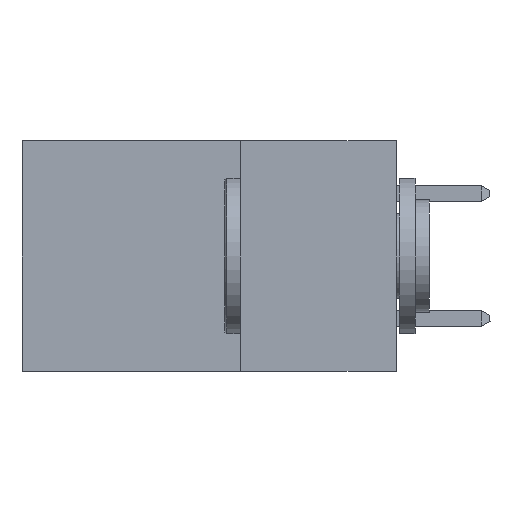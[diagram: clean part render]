
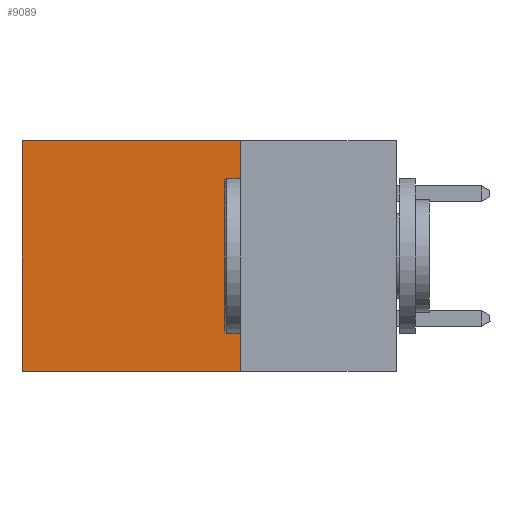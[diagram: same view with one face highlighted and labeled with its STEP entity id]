
A CAD part, left-side view. The second image highlights one B-rep face of the part: STEP entity #9089.
In plain terms, the highlighted planar face has unit normal (-1, 0, 0).
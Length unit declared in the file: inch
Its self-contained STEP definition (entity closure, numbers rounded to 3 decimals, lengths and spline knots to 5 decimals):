
#86 = ORIENTED_EDGE ( 'NONE', *, *, #2505, .F. ) ;
#507 = PLANE ( 'NONE',  #6340 ) ;
#797 = VECTOR ( 'NONE', #9953, 39.37008 ) ;
#891 = CARTESIAN_POINT ( 'NONE',  ( 0.2615, 0.25, -0.37 ) ) ;
#1397 = EDGE_CURVE ( 'NONE', #5189, #5558, #2477, .T. ) ;
#2044 = DIRECTION ( 'NONE',  ( 1., 0., 0. ) ) ;
#2215 = VECTOR ( 'NONE', #5669, 39.37008 ) ;
#2477 = LINE ( 'NONE', #4899, #2215 ) ;
#2505 = EDGE_CURVE ( 'NONE', #5189, #9576, #9101, .T. ) ;
#2617 = LINE ( 'NONE', #4548, #8103 ) ;
#2739 = EDGE_CURVE ( 'NONE', #9576, #9796, #5337, .T. ) ;
#3439 = ORIENTED_EDGE ( 'NONE', *, *, #1397, .T. ) ;
#3750 = VECTOR ( 'NONE', #9432, 39.37008 ) ;
#4528 = CARTESIAN_POINT ( 'NONE',  ( 0.2615, 0.25, -0.37 ) ) ;
#4548 = CARTESIAN_POINT ( 'NONE',  ( 0.2615, 0.6, -0.37 ) ) ;
#4899 = CARTESIAN_POINT ( 'NONE',  ( 0.2615, 0.25, 0. ) ) ;
#5189 = VERTEX_POINT ( 'NONE', #6603 ) ;
#5337 = LINE ( 'NONE', #8490, #797 ) ;
#5410 = DIRECTION ( 'NONE',  ( 0., 0., -1. ) ) ;
#5476 = FACE_OUTER_BOUND ( 'NONE', #10094, .T. ) ;
#5558 = VERTEX_POINT ( 'NONE', #8552 ) ;
#5606 = ORIENTED_EDGE ( 'NONE', *, *, #7012, .T. ) ;
#5669 = DIRECTION ( 'NONE',  ( 0., 1., 0. ) ) ;
#6340 = AXIS2_PLACEMENT_3D ( 'NONE', #10414, #2044, #9556 ) ;
#6603 = CARTESIAN_POINT ( 'NONE',  ( 0.2615, 0.25, 0. ) ) ;
#6904 = ORIENTED_EDGE ( 'NONE', *, *, #2739, .F. ) ;
#7012 = EDGE_CURVE ( 'NONE', #5558, #9796, #2617, .T. ) ;
#8103 = VECTOR ( 'NONE', #5410, 39.37008 ) ;
#8490 = CARTESIAN_POINT ( 'NONE',  ( 0.2615, 0.25, -0.37 ) ) ;
#8552 = CARTESIAN_POINT ( 'NONE',  ( 0.2615, 0.6, 0. ) ) ;
#9089 = ADVANCED_FACE ( 'NONE', ( #5476 ), #507, .F. ) ;
#9101 = LINE ( 'NONE', #4528, #3750 ) ;
#9432 = DIRECTION ( 'NONE',  ( 0., 0., -1. ) ) ;
#9556 = DIRECTION ( 'NONE',  ( 0., 0., -1. ) ) ;
#9576 = VERTEX_POINT ( 'NONE', #891 ) ;
#9796 = VERTEX_POINT ( 'NONE', #10494 ) ;
#9953 = DIRECTION ( 'NONE',  ( 0., 1., 0. ) ) ;
#10094 = EDGE_LOOP ( 'NONE', ( #5606, #6904, #86, #3439 ) ) ;
#10414 = CARTESIAN_POINT ( 'NONE',  ( 0.2615, 0.25, -0.37 ) ) ;
#10494 = CARTESIAN_POINT ( 'NONE',  ( 0.2615, 0.6, -0.37 ) ) ;
